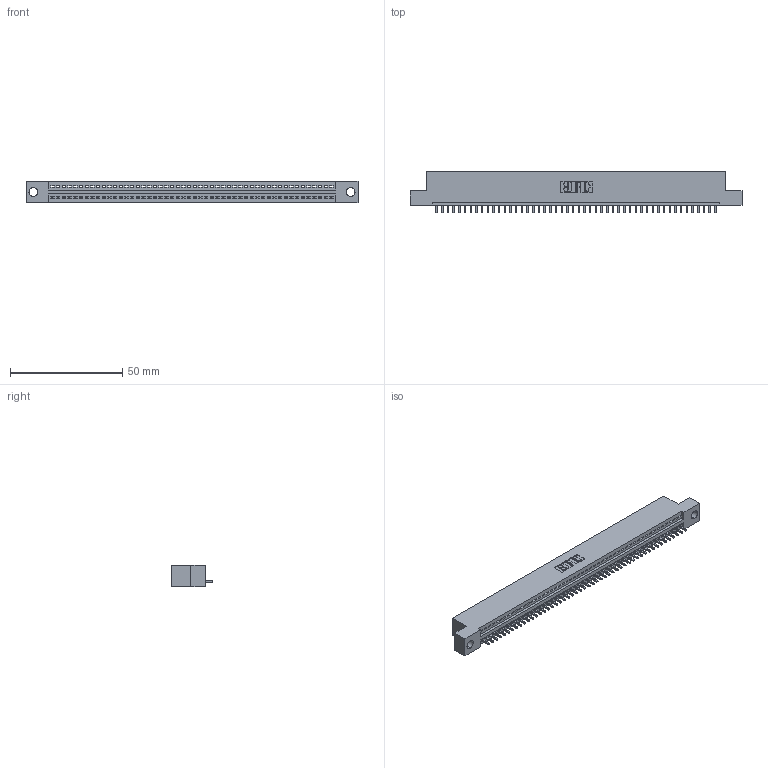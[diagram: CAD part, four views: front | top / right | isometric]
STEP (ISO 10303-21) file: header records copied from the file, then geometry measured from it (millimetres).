
FILE_DESCRIPTION (( 'STEP AP203' ), '1' );
FILE_NAME ('345-050-521-104.STEP', '2021-05-26T15:20:19', ( '' ), ( '' ), 'SwSTEP 2.0', 'SolidWorks 2020', '' );
FILE_SCHEMA (( 'CONFIG_CONTROL_DESIGN' ));
Length unit declared in the file: inch
Products named in the file (3): 345-050-521-104; 345-292-001_345-293-121; 345 Part_Flush Mounting Lugs - 0.156 Dia-TI
Assembly tree (51 placements, depth 2):
  345-050-521-104
    345 Part_Flush Mounting Lugs - 0.156 Dia-TI
    345-292-001_345-293-121  x50
Bounding box: 148.21 x 18.72 x 9.4 mm (x, y, z)
Volume: 13894.4 mm3; surface area: 17859.2 mm2
Topology: 51 solids, 51 shells, 3040 faces, 9177 edges, 6050 vertices
Faces by surface type: plane 2094, cylinder 946
Entity records: 36991 total; most frequent: CARTESIAN_POINT 6416, ORIENTED_EDGE 6398, DIRECTION 5591, EDGE_CURVE 3199, VECTOR 2867, LINE 2867, VERTEX_POINT 2130, AXIS2_PLACEMENT_3D 1362
